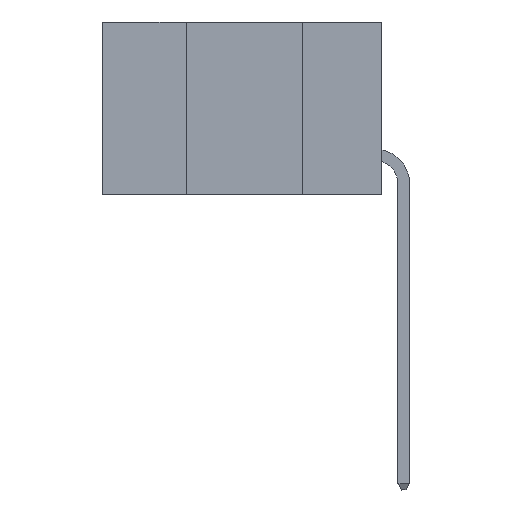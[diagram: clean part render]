
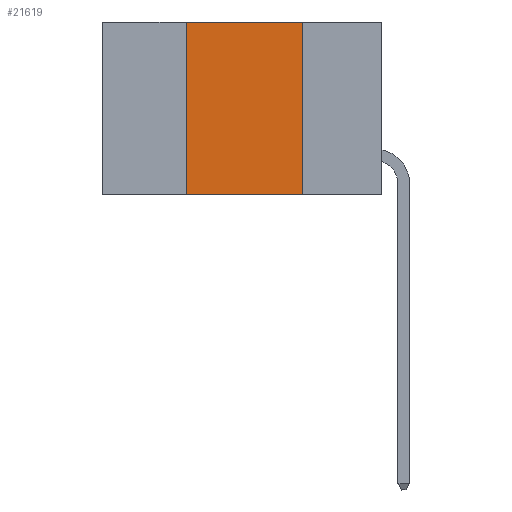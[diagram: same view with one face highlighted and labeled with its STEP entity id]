
A CAD part, left-side view. The second image highlights one B-rep face of the part: STEP entity #21619.
In plain terms, the highlighted planar face has unit normal (-1, 0, 0).
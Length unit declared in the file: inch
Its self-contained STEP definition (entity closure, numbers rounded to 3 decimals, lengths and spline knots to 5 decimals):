
#778 = VERTEX_POINT ( 'NONE', #22655 ) ;
#797 = EDGE_CURVE ( 'NONE', #22795, #778, #2307, .T. ) ;
#1483 = VECTOR ( 'NONE', #36924, 39.37008 ) ;
#2307 = LINE ( 'NONE', #33955, #33713 ) ;
#3023 = VERTEX_POINT ( 'NONE', #21100 ) ;
#4472 = DIRECTION ( 'NONE',  ( 0., -1., 0. ) ) ;
#4935 = DIRECTION ( 'NONE',  ( 0., 0., -1. ) ) ;
#5144 = EDGE_CURVE ( 'NONE', #46035, #22795, #10120, .T. ) ;
#5642 = CARTESIAN_POINT ( 'NONE',  ( 0., 0.6, 0. ) ) ;
#6402 = CARTESIAN_POINT ( 'NONE',  ( 0., 0.42, 0. ) ) ;
#10120 = LINE ( 'NONE', #33063, #1483 ) ;
#10151 = ORIENTED_EDGE ( 'NONE', *, *, #23254, .T. ) ;
#10773 = ORIENTED_EDGE ( 'NONE', *, *, #797, .F. ) ;
#15082 = AXIS2_PLACEMENT_3D ( 'NONE', #5642, #27323, #38472 ) ;
#15489 = VECTOR ( 'NONE', #25528, 39.37008 ) ;
#16623 = LINE ( 'NONE', #6402, #15489 ) ;
#16678 = LINE ( 'NONE', #29664, #30928 ) ;
#18660 = CARTESIAN_POINT ( 'NONE',  ( 0., 0.17, 0. ) ) ;
#21100 = CARTESIAN_POINT ( 'NONE',  ( 0., 0.42, -0.37 ) ) ;
#21619 = ADVANCED_FACE ( 'NONE', ( #22572 ), #45819, .F. ) ;
#22197 = CARTESIAN_POINT ( 'NONE',  ( 0., 0.42, 0. ) ) ;
#22572 = FACE_OUTER_BOUND ( 'NONE', #42982, .T. ) ;
#22655 = CARTESIAN_POINT ( 'NONE',  ( 0., 0.17, -0.37 ) ) ;
#22795 = VERTEX_POINT ( 'NONE', #18660 ) ;
#23254 = EDGE_CURVE ( 'NONE', #3023, #778, #16678, .T. ) ;
#24792 = ORIENTED_EDGE ( 'NONE', *, *, #5144, .F. ) ;
#25528 = DIRECTION ( 'NONE',  ( 0., 0., 1. ) ) ;
#27323 = DIRECTION ( 'NONE',  ( 1., 0., 0. ) ) ;
#28235 = ORIENTED_EDGE ( 'NONE', *, *, #34340, .F. ) ;
#29664 = CARTESIAN_POINT ( 'NONE',  ( 0., 0.6, -0.37 ) ) ;
#30928 = VECTOR ( 'NONE', #4472, 39.37008 ) ;
#33063 = CARTESIAN_POINT ( 'NONE',  ( 0., 0.6, 0. ) ) ;
#33713 = VECTOR ( 'NONE', #4935, 39.37008 ) ;
#33955 = CARTESIAN_POINT ( 'NONE',  ( 0., 0.17, 0. ) ) ;
#34340 = EDGE_CURVE ( 'NONE', #3023, #46035, #16623, .T. ) ;
#36924 = DIRECTION ( 'NONE',  ( 0., -1., 0. ) ) ;
#38472 = DIRECTION ( 'NONE',  ( 0., 0., -1. ) ) ;
#42982 = EDGE_LOOP ( 'NONE', ( #10773, #24792, #28235, #10151 ) ) ;
#45819 = PLANE ( 'NONE',  #15082 ) ;
#46035 = VERTEX_POINT ( 'NONE', #22197 ) ;
